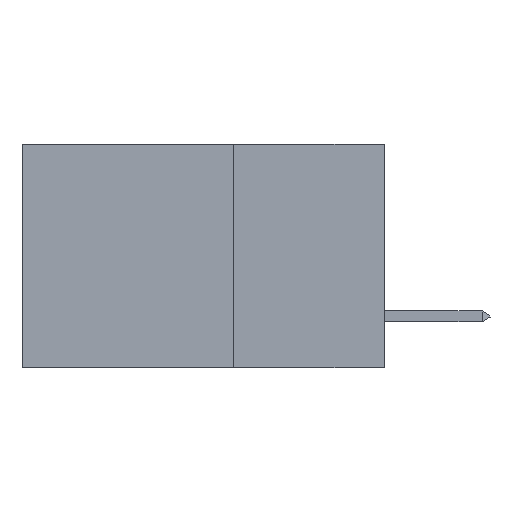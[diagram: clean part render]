
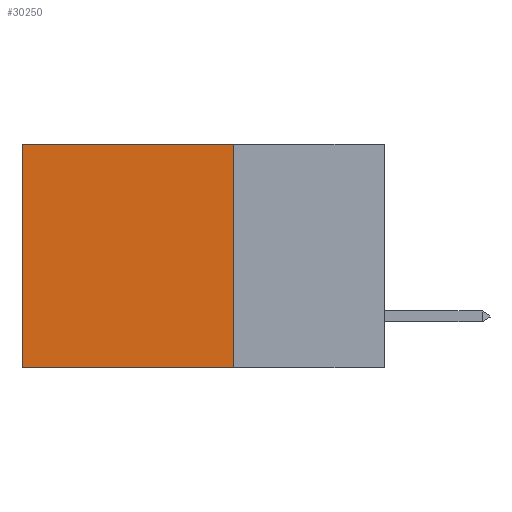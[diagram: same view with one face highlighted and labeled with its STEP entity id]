
A CAD part, left-side view. The second image highlights one B-rep face of the part: STEP entity #30250.
In plain terms, the highlighted planar face has unit normal (-1, 0, 0).
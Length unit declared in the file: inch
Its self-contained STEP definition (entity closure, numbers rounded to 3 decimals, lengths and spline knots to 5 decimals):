
#2740 = EDGE_CURVE ( 'NONE', #27333, #16183, #29340, .T. ) ;
#3115 = DIRECTION ( 'NONE',  ( 0., 0., -1. ) ) ;
#3586 = VECTOR ( 'NONE', #16533, 39.37008 ) ;
#3931 = VERTEX_POINT ( 'NONE', #39634 ) ;
#4132 = LINE ( 'NONE', #9263, #3586 ) ;
#5337 = DIRECTION ( 'NONE',  ( 0., 1., 0. ) ) ;
#6035 = EDGE_CURVE ( 'NONE', #25339, #27333, #35245, .T. ) ;
#9263 = CARTESIAN_POINT ( 'NONE',  ( 0.2875, 0.25, -0.37 ) ) ;
#11667 = AXIS2_PLACEMENT_3D ( 'NONE', #23555, #16636, #3115 ) ;
#16183 = VERTEX_POINT ( 'NONE', #34445 ) ;
#16533 = DIRECTION ( 'NONE',  ( 0., 1., 0. ) ) ;
#16636 = DIRECTION ( 'NONE',  ( 1., 0., 0. ) ) ;
#21173 = EDGE_CURVE ( 'NONE', #25339, #3931, #30806, .T. ) ;
#22169 = DIRECTION ( 'NONE',  ( 0., 0., -1. ) ) ;
#23098 = ORIENTED_EDGE ( 'NONE', *, *, #21173, .F. ) ;
#23555 = CARTESIAN_POINT ( 'NONE',  ( 0.2875, 0.25, 0. ) ) ;
#25339 = VERTEX_POINT ( 'NONE', #28237 ) ;
#26339 = VECTOR ( 'NONE', #5337, 39.37008 ) ;
#26613 = PLANE ( 'NONE',  #11667 ) ;
#27333 = VERTEX_POINT ( 'NONE', #29937 ) ;
#27660 = VECTOR ( 'NONE', #36739, 39.37008 ) ;
#27793 = VECTOR ( 'NONE', #22169, 39.37008 ) ;
#28237 = CARTESIAN_POINT ( 'NONE',  ( 0.2875, 0.25, 0. ) ) ;
#28465 = EDGE_CURVE ( 'NONE', #3931, #16183, #4132, .T. ) ;
#28835 = FACE_OUTER_BOUND ( 'NONE', #40951, .T. ) ;
#29340 = LINE ( 'NONE', #42237, #27793 ) ;
#29937 = CARTESIAN_POINT ( 'NONE',  ( 0.2875, 0.6, 0. ) ) ;
#30250 = ADVANCED_FACE ( 'NONE', ( #28835 ), #26613, .F. ) ;
#30806 = LINE ( 'NONE', #43189, #27660 ) ;
#31633 = ORIENTED_EDGE ( 'NONE', *, *, #2740, .T. ) ;
#34445 = CARTESIAN_POINT ( 'NONE',  ( 0.2875, 0.6, -0.37 ) ) ;
#35245 = LINE ( 'NONE', #37964, #26339 ) ;
#36739 = DIRECTION ( 'NONE',  ( 0., 0., -1. ) ) ;
#37964 = CARTESIAN_POINT ( 'NONE',  ( 0.2875, 0.25, 0. ) ) ;
#38250 = ORIENTED_EDGE ( 'NONE', *, *, #6035, .T. ) ;
#39634 = CARTESIAN_POINT ( 'NONE',  ( 0.2875, 0.25, -0.37 ) ) ;
#40951 = EDGE_LOOP ( 'NONE', ( #31633, #42965, #23098, #38250 ) ) ;
#42237 = CARTESIAN_POINT ( 'NONE',  ( 0.2875, 0.6, 0. ) ) ;
#42965 = ORIENTED_EDGE ( 'NONE', *, *, #28465, .F. ) ;
#43189 = CARTESIAN_POINT ( 'NONE',  ( 0.2875, 0.25, 0. ) ) ;
